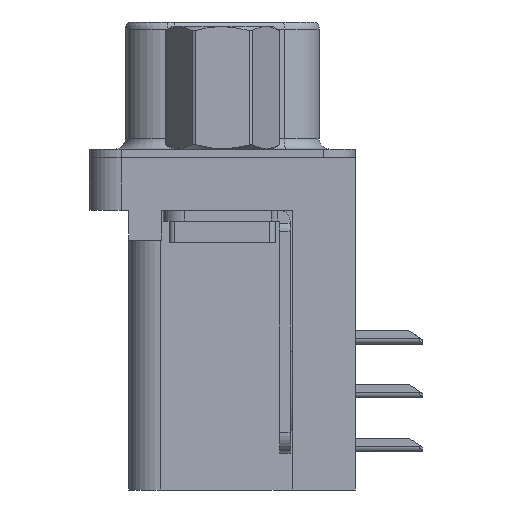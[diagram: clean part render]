
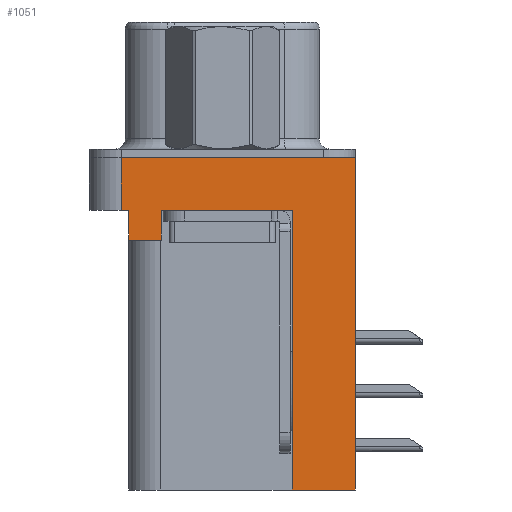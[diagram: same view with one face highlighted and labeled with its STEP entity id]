
A CAD part, left-side view. The second image highlights one B-rep face of the part: STEP entity #1051.
In plain terms, the highlighted planar face has unit normal (-1, 0, 0).
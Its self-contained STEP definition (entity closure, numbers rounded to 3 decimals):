
#1051 = ADVANCED_FACE ( 'NONE', ( #20315 ), #19256, .T. ) ;
#1825 = VERTEX_POINT ( 'NONE', #22005 ) ;
#1883 = CARTESIAN_POINT ( 'NONE',  ( -2.935, 4.425, -3.9 ) ) ;
#2186 = EDGE_CURVE ( 'NONE', #4132, #9068, #27141, .T. ) ;
#2229 = AXIS2_PLACEMENT_3D ( 'NONE', #22883, #22200, #22143 ) ;
#3225 = CARTESIAN_POINT ( 'NONE',  ( -2.935, 2.895, -2.5 ) ) ;
#3822 = CARTESIAN_POINT ( 'NONE',  ( -2.935, -3.295, -15.7 ) ) ;
#3986 = CARTESIAN_POINT ( 'NONE',  ( -2.935, -6.275, 0. ) ) ;
#4132 = VERTEX_POINT ( 'NONE', #13663 ) ;
#4660 = DIRECTION ( 'NONE',  ( 0., 0., 1. ) ) ;
#4795 = VECTOR ( 'NONE', #12873, 1000. ) ;
#4832 = ORIENTED_EDGE ( 'NONE', *, *, #23375, .F. ) ;
#5020 = CARTESIAN_POINT ( 'NONE',  ( -2.935, -6.275, -2.5 ) ) ;
#5402 = ORIENTED_EDGE ( 'NONE', *, *, #9534, .T. ) ;
#5471 = LINE ( 'NONE', #5020, #29284 ) ;
#5573 = VECTOR ( 'NONE', #15634, 1000. ) ;
#5609 = VECTOR ( 'NONE', #28692, 1000. ) ;
#5760 = LINE ( 'NONE', #13516, #29560 ) ;
#5963 = VERTEX_POINT ( 'NONE', #22397 ) ;
#6164 = LINE ( 'NONE', #22697, #18326 ) ;
#7314 = ORIENTED_EDGE ( 'NONE', *, *, #26473, .F. ) ;
#7778 = ORIENTED_EDGE ( 'NONE', *, *, #2186, .T. ) ;
#7785 = LINE ( 'NONE', #10238, #5609 ) ;
#7861 = VERTEX_POINT ( 'NONE', #12343 ) ;
#8463 = DIRECTION ( 'NONE',  ( 0., 0., 1. ) ) ;
#8780 = ORIENTED_EDGE ( 'NONE', *, *, #22942, .F. ) ;
#9017 = DIRECTION ( 'NONE',  ( 0., 0., 1. ) ) ;
#9068 = VERTEX_POINT ( 'NONE', #3225 ) ;
#9534 = EDGE_CURVE ( 'NONE', #20304, #1825, #5471, .T. ) ;
#9665 = DIRECTION ( 'NONE',  ( 0., 0., 1. ) ) ;
#10238 = CARTESIAN_POINT ( 'NONE',  ( -2.935, -6.275, -2.5 ) ) ;
#11688 = CARTESIAN_POINT ( 'NONE',  ( -2.935, 4.425, -3.9 ) ) ;
#11803 = VERTEX_POINT ( 'NONE', #13234 ) ;
#12343 = CARTESIAN_POINT ( 'NONE',  ( -2.935, 4.775, -2.5 ) ) ;
#12771 = CARTESIAN_POINT ( 'NONE',  ( -2.935, -6.275, -2.5 ) ) ;
#12873 = DIRECTION ( 'NONE',  ( 0., -1., 0. ) ) ;
#13061 = VECTOR ( 'NONE', #8463, 1000. ) ;
#13234 = CARTESIAN_POINT ( 'NONE',  ( -2.935, 4.775, 0. ) ) ;
#13516 = CARTESIAN_POINT ( 'NONE',  ( -2.935, 4.775, -2.5 ) ) ;
#13663 = CARTESIAN_POINT ( 'NONE',  ( -2.935, 2.895, -3.9 ) ) ;
#13986 = DIRECTION ( 'NONE',  ( 0., 1., 0. ) ) ;
#14883 = VECTOR ( 'NONE', #4660, 1000. ) ;
#15157 = CARTESIAN_POINT ( 'NONE',  ( -2.935, -3.295, -15.7 ) ) ;
#15255 = VERTEX_POINT ( 'NONE', #18339 ) ;
#15587 = EDGE_CURVE ( 'NONE', #7861, #15255, #29342, .T. ) ;
#15634 = DIRECTION ( 'NONE',  ( 0., 0., 1. ) ) ;
#16266 = VECTOR ( 'NONE', #13986, 1000. ) ;
#17204 = EDGE_CURVE ( 'NONE', #20304, #28926, #6164, .T. ) ;
#18326 = VECTOR ( 'NONE', #20359, 1000. ) ;
#18339 = CARTESIAN_POINT ( 'NONE',  ( -2.935, 4.425, -2.5 ) ) ;
#19112 = LINE ( 'NONE', #3822, #13061 ) ;
#19256 = PLANE ( 'NONE',  #2229 ) ;
#20035 = DIRECTION ( 'NONE',  ( 0., -1., 0. ) ) ;
#20304 = VERTEX_POINT ( 'NONE', #23841 ) ;
#20315 = FACE_OUTER_BOUND ( 'NONE', #27508, .T. ) ;
#20359 = DIRECTION ( 'NONE',  ( 0., 1., 0. ) ) ;
#20630 = VERTEX_POINT ( 'NONE', #22602 ) ;
#21076 = EDGE_CURVE ( 'NONE', #9068, #5963, #7785, .T. ) ;
#21709 = LINE ( 'NONE', #3986, #27123 ) ;
#22005 = CARTESIAN_POINT ( 'NONE',  ( -2.935, -6.275, 0. ) ) ;
#22143 = DIRECTION ( 'NONE',  ( 0., 0., 1. ) ) ;
#22200 = DIRECTION ( 'NONE',  ( -1., 0., 0. ) ) ;
#22397 = CARTESIAN_POINT ( 'NONE',  ( -2.935, -3.295, -2.5 ) ) ;
#22421 = LINE ( 'NONE', #11688, #16266 ) ;
#22602 = CARTESIAN_POINT ( 'NONE',  ( -2.935, 4.425, -3.9 ) ) ;
#22697 = CARTESIAN_POINT ( 'NONE',  ( -2.935, -3.295, -15.7 ) ) ;
#22883 = CARTESIAN_POINT ( 'NONE',  ( -2.935, -6.275, -2.5 ) ) ;
#22942 = EDGE_CURVE ( 'NONE', #4132, #20630, #22421, .T. ) ;
#23375 = EDGE_CURVE ( 'NONE', #28926, #5963, #19112, .T. ) ;
#23841 = CARTESIAN_POINT ( 'NONE',  ( -2.935, -6.275, -15.7 ) ) ;
#24228 = CARTESIAN_POINT ( 'NONE',  ( -2.935, 2.895, -3.9 ) ) ;
#24914 = EDGE_CURVE ( 'NONE', #20630, #15255, #29374, .T. ) ;
#25480 = ORIENTED_EDGE ( 'NONE', *, *, #17204, .F. ) ;
#26206 = ORIENTED_EDGE ( 'NONE', *, *, #15587, .T. ) ;
#26473 = EDGE_CURVE ( 'NONE', #11803, #1825, #21709, .T. ) ;
#27123 = VECTOR ( 'NONE', #20035, 1000. ) ;
#27141 = LINE ( 'NONE', #24228, #14883 ) ;
#27508 = EDGE_LOOP ( 'NONE', ( #7314, #28416, #26206, #28358, #8780, #7778, #28145, #4832, #25480, #5402 ) ) ;
#28145 = ORIENTED_EDGE ( 'NONE', *, *, #21076, .T. ) ;
#28358 = ORIENTED_EDGE ( 'NONE', *, *, #24914, .F. ) ;
#28416 = ORIENTED_EDGE ( 'NONE', *, *, #29633, .F. ) ;
#28692 = DIRECTION ( 'NONE',  ( 0., -1., 0. ) ) ;
#28926 = VERTEX_POINT ( 'NONE', #15157 ) ;
#29284 = VECTOR ( 'NONE', #9665, 1000. ) ;
#29342 = LINE ( 'NONE', #12771, #4795 ) ;
#29374 = LINE ( 'NONE', #1883, #5573 ) ;
#29560 = VECTOR ( 'NONE', #9017, 1000. ) ;
#29633 = EDGE_CURVE ( 'NONE', #7861, #11803, #5760, .T. ) ;
